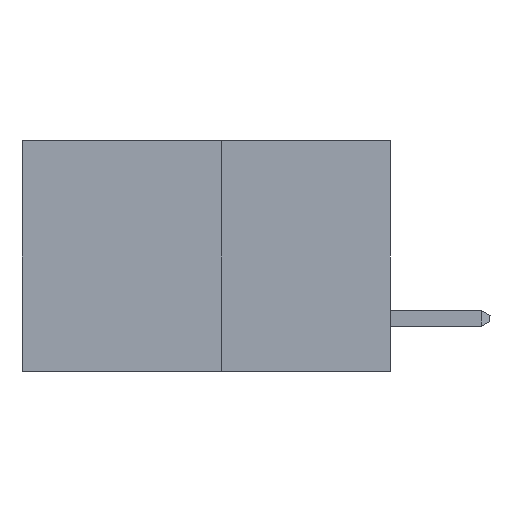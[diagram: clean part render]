
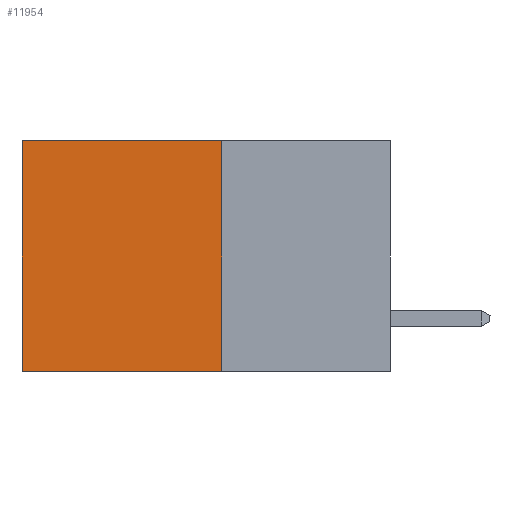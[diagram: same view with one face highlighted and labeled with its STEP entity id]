
A CAD part, left-side view. The second image highlights one B-rep face of the part: STEP entity #11954.
In plain terms, the highlighted planar face has unit normal (-1, 0, 0).
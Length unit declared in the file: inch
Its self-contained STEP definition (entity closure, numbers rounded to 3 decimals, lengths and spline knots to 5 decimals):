
#1459 = CARTESIAN_POINT ( 'NONE',  ( 0.277, 0.27, 0. ) ) ;
#1627 = EDGE_CURVE ( 'NONE', #5527, #6022, #17411, .T. ) ;
#1684 = EDGE_CURVE ( 'NONE', #3176, #6022, #16923, .T. ) ;
#2246 = CARTESIAN_POINT ( 'NONE',  ( 0.277, 0.27, -0.37 ) ) ;
#2296 = CARTESIAN_POINT ( 'NONE',  ( 0.277, 0.27, 0. ) ) ;
#2918 = EDGE_CURVE ( 'NONE', #4291, #5527, #5343, .T. ) ;
#3176 = VERTEX_POINT ( 'NONE', #14029 ) ;
#3532 = LINE ( 'NONE', #15605, #15530 ) ;
#3684 = ORIENTED_EDGE ( 'NONE', *, *, #1684, .F. ) ;
#3916 = ORIENTED_EDGE ( 'NONE', *, *, #2918, .T. ) ;
#4291 = VERTEX_POINT ( 'NONE', #2296 ) ;
#4361 = CARTESIAN_POINT ( 'NONE',  ( 0.277, 0.59, 0. ) ) ;
#4880 = VECTOR ( 'NONE', #8181, 39.37008 ) ;
#5343 = LINE ( 'NONE', #1459, #4880 ) ;
#5527 = VERTEX_POINT ( 'NONE', #4361 ) ;
#6022 = VERTEX_POINT ( 'NONE', #12537 ) ;
#6778 = EDGE_CURVE ( 'NONE', #4291, #3176, #3532, .T. ) ;
#8099 = VECTOR ( 'NONE', #10893, 39.37008 ) ;
#8181 = DIRECTION ( 'NONE',  ( 0., 1., 0. ) ) ;
#8255 = DIRECTION ( 'NONE',  ( 1., 0., 0. ) ) ;
#9064 = VECTOR ( 'NONE', #15900, 39.37008 ) ;
#10893 = DIRECTION ( 'NONE',  ( 0., 1., 0. ) ) ;
#11160 = DIRECTION ( 'NONE',  ( 0., 0., -1. ) ) ;
#11954 = ADVANCED_FACE ( 'NONE', ( #17435 ), #16087, .F. ) ;
#12537 = CARTESIAN_POINT ( 'NONE',  ( 0.277, 0.59, -0.37 ) ) ;
#13909 = ORIENTED_EDGE ( 'NONE', *, *, #1627, .T. ) ;
#14029 = CARTESIAN_POINT ( 'NONE',  ( 0.277, 0.27, -0.37 ) ) ;
#14457 = ORIENTED_EDGE ( 'NONE', *, *, #6778, .F. ) ;
#15275 = CARTESIAN_POINT ( 'NONE',  ( 0.277, 0.59, -0.37 ) ) ;
#15530 = VECTOR ( 'NONE', #11160, 39.37008 ) ;
#15605 = CARTESIAN_POINT ( 'NONE',  ( 0.277, 0.27, -0.37 ) ) ;
#15900 = DIRECTION ( 'NONE',  ( 0., 0., -1. ) ) ;
#16087 = PLANE ( 'NONE',  #17456 ) ;
#16923 = LINE ( 'NONE', #2246, #8099 ) ;
#17411 = LINE ( 'NONE', #15275, #9064 ) ;
#17435 = FACE_OUTER_BOUND ( 'NONE', #20019, .T. ) ;
#17456 = AXIS2_PLACEMENT_3D ( 'NONE', #17635, #8255, #19212 ) ;
#17635 = CARTESIAN_POINT ( 'NONE',  ( 0.277, 0.27, -0.37 ) ) ;
#19212 = DIRECTION ( 'NONE',  ( 0., 0., -1. ) ) ;
#20019 = EDGE_LOOP ( 'NONE', ( #13909, #3684, #14457, #3916 ) ) ;
